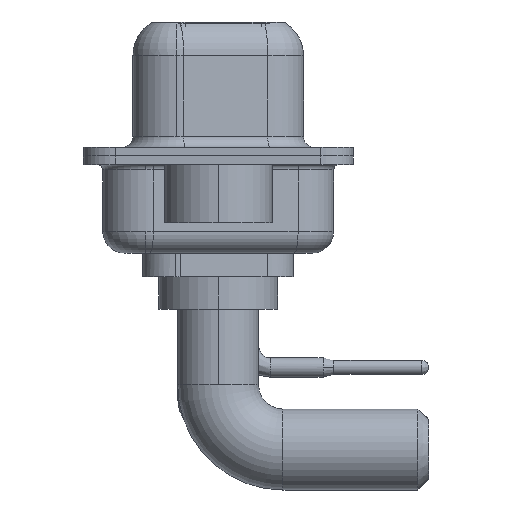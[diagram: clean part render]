
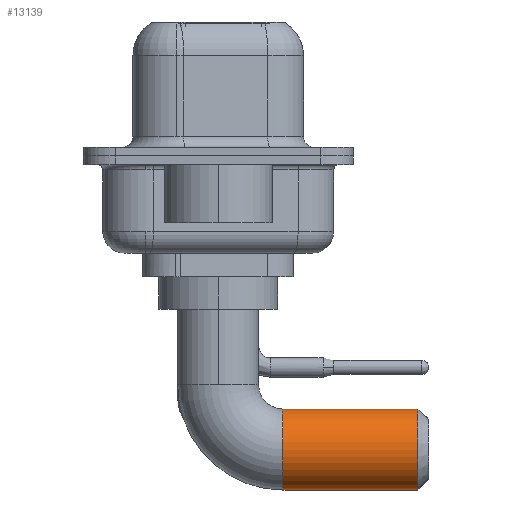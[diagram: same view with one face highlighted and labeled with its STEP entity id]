
A CAD part, left-side view. The second image highlights one B-rep face of the part: STEP entity #13139.
In plain terms, the highlighted cylindrical face has radius 1.875 mm (diameter 3.75 mm), a partial arc.
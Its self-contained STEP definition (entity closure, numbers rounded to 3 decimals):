
#907 = CARTESIAN_POINT ( 'NONE',  ( 0., -9.25, -6.5 ) ) ;
#1024 = EDGE_CURVE ( 'NONE', #11406, #15431, #4537, .T. ) ;
#1389 = DIRECTION ( 'NONE',  ( 0., 0., -1. ) ) ;
#1916 = DIRECTION ( 'NONE',  ( 0., -1., 0. ) ) ;
#2390 = DIRECTION ( 'NONE',  ( 0., 0., -1. ) ) ;
#3413 = VECTOR ( 'NONE', #1916, 1000. ) ;
#3442 = CARTESIAN_POINT ( 'NONE',  ( 0., -3., -8.375 ) ) ;
#3714 = EDGE_CURVE ( 'NONE', #4194, #15431, #11063, .T. ) ;
#3725 = CARTESIAN_POINT ( 'NONE',  ( 0., -9.25, -4.625 ) ) ;
#3765 = FACE_OUTER_BOUND ( 'NONE', #4159, .T. ) ;
#4159 = EDGE_LOOP ( 'NONE', ( #11045, #4611, #6997, #5282 ) ) ;
#4194 = VERTEX_POINT ( 'NONE', #4816 ) ;
#4537 = LINE ( 'NONE', #8912, #3413 ) ;
#4611 = ORIENTED_EDGE ( 'NONE', *, *, #16352, .T. ) ;
#4816 = CARTESIAN_POINT ( 'NONE',  ( 0., -9.25, -8.375 ) ) ;
#5282 = ORIENTED_EDGE ( 'NONE', *, *, #3714, .T. ) ;
#5416 = CIRCLE ( 'NONE', #14075, 1.875 ) ;
#5745 = AXIS2_PLACEMENT_3D ( 'NONE', #907, #17018, #2390 ) ;
#6265 = CARTESIAN_POINT ( 'NONE',  ( 0., -3., -4.625 ) ) ;
#6808 = DIRECTION ( 'NONE',  ( 0., -1., 0. ) ) ;
#6848 = EDGE_CURVE ( 'NONE', #12523, #4194, #16764, .T. ) ;
#6997 = ORIENTED_EDGE ( 'NONE', *, *, #6848, .T. ) ;
#8912 = CARTESIAN_POINT ( 'NONE',  ( 0., -3., -4.625 ) ) ;
#11045 = ORIENTED_EDGE ( 'NONE', *, *, #1024, .F. ) ;
#11063 = CIRCLE ( 'NONE', #5745, 1.875 ) ;
#11406 = VERTEX_POINT ( 'NONE', #6265 ) ;
#12096 = DIRECTION ( 'NONE',  ( -1., 0., 0. ) ) ;
#12523 = VERTEX_POINT ( 'NONE', #15698 ) ;
#13139 = ADVANCED_FACE ( 'NONE', ( #3765 ), #15766, .T. ) ;
#14075 = AXIS2_PLACEMENT_3D ( 'NONE', #14734, #14815, #12096 ) ;
#14734 = CARTESIAN_POINT ( 'NONE',  ( 0., -3., -6.5 ) ) ;
#14815 = DIRECTION ( 'NONE',  ( 0., -1., 0. ) ) ;
#15431 = VERTEX_POINT ( 'NONE', #3725 ) ;
#15628 = DIRECTION ( 'NONE',  ( 0., -1., 0. ) ) ;
#15698 = CARTESIAN_POINT ( 'NONE',  ( 0., -3., -8.375 ) ) ;
#15712 = AXIS2_PLACEMENT_3D ( 'NONE', #16115, #6808, #1389 ) ;
#15766 = CYLINDRICAL_SURFACE ( 'NONE', #15712, 1.875 ) ;
#16115 = CARTESIAN_POINT ( 'NONE',  ( 0., -3., -6.5 ) ) ;
#16352 = EDGE_CURVE ( 'NONE', #11406, #12523, #5416, .T. ) ;
#16697 = VECTOR ( 'NONE', #15628, 1000. ) ;
#16764 = LINE ( 'NONE', #3442, #16697 ) ;
#17018 = DIRECTION ( 'NONE',  ( 0., 1., 0. ) ) ;
